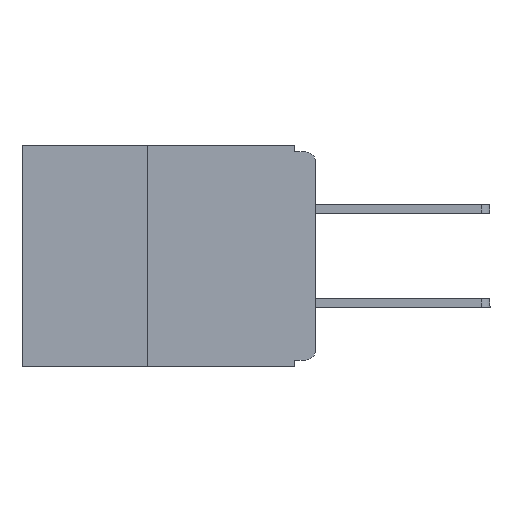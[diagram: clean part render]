
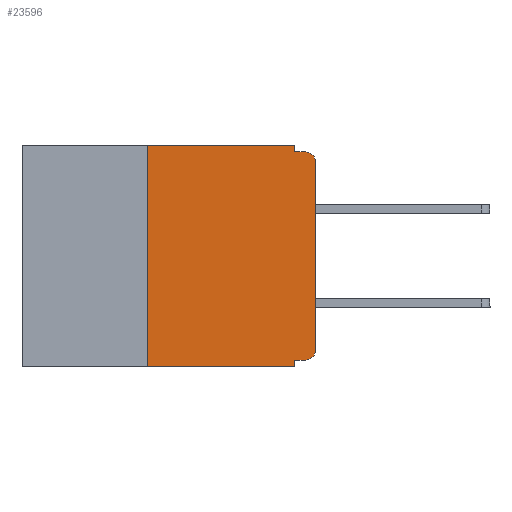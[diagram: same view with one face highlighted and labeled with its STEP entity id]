
A CAD part, left-side view. The second image highlights one B-rep face of the part: STEP entity #23596.
In plain terms, the highlighted planar face has unit normal (-1, 0, 0).
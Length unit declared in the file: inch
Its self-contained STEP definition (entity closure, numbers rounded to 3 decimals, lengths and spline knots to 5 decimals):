
#264 = EDGE_CURVE ( 'NONE', #24126, #7658, #23924, .T. ) ;
#312 = ORIENTED_EDGE ( 'NONE', *, *, #5832, .F. ) ;
#1313 = DIRECTION ( 'NONE',  ( 0., -1., 0. ) ) ;
#1519 = ORIENTED_EDGE ( 'NONE', *, *, #21155, .T. ) ;
#1641 = LINE ( 'NONE', #26766, #6741 ) ;
#2126 = EDGE_CURVE ( 'NONE', #22925, #6233, #27481, .T. ) ;
#2175 = ORIENTED_EDGE ( 'NONE', *, *, #25686, .F. ) ;
#2675 = CARTESIAN_POINT ( 'NONE',  ( 0., 0.015, -0.305 ) ) ;
#2694 = ORIENTED_EDGE ( 'NONE', *, *, #17311, .F. ) ;
#3103 = ORIENTED_EDGE ( 'NONE', *, *, #22706, .T. ) ;
#3152 = ORIENTED_EDGE ( 'NONE', *, *, #14555, .T. ) ;
#3421 = CARTESIAN_POINT ( 'NONE',  ( 0., 0., -0.305 ) ) ;
#3519 = CARTESIAN_POINT ( 'NONE',  ( 0., 0.031, -0.32 ) ) ;
#3711 = VERTEX_POINT ( 'NONE', #3519 ) ;
#4563 = DIRECTION ( 'NONE',  ( 0., 0., -1. ) ) ;
#4694 = CARTESIAN_POINT ( 'NONE',  ( 0., 0., -0.025 ) ) ;
#4832 = DIRECTION ( 'NONE',  ( 0., 0., -1. ) ) ;
#4986 = LINE ( 'NONE', #14463, #15992 ) ;
#5126 = ORIENTED_EDGE ( 'NONE', *, *, #20510, .F. ) ;
#5166 = VECTOR ( 'NONE', #14456, 39.37008 ) ;
#5707 = VECTOR ( 'NONE', #16219, 39.37008 ) ;
#5832 = EDGE_CURVE ( 'NONE', #23705, #10160, #15461, .T. ) ;
#6147 = CARTESIAN_POINT ( 'NONE',  ( 0., 0.25, -0.33 ) ) ;
#6233 = VERTEX_POINT ( 'NONE', #15600 ) ;
#6489 = VECTOR ( 'NONE', #25533, 39.37008 ) ;
#6550 = VERTEX_POINT ( 'NONE', #25217 ) ;
#6741 = VECTOR ( 'NONE', #18208, 39.37008 ) ;
#7175 = CARTESIAN_POINT ( 'NONE',  ( 0., 0.015, -0.025 ) ) ;
#7658 = VERTEX_POINT ( 'NONE', #4694 ) ;
#8170 = AXIS2_PLACEMENT_3D ( 'NONE', #2675, #17972, #4832 ) ;
#9197 = LINE ( 'NONE', #25203, #20206 ) ;
#9242 = CIRCLE ( 'NONE', #8170, 0.015 ) ;
#9347 = DIRECTION ( 'NONE',  ( 0., 0., -1. ) ) ;
#9460 = CARTESIAN_POINT ( 'NONE',  ( 0., 0.031, 0. ) ) ;
#9952 = CARTESIAN_POINT ( 'NONE',  ( 0., 0.031, 0. ) ) ;
#10160 = VERTEX_POINT ( 'NONE', #26424 ) ;
#10274 = VERTEX_POINT ( 'NONE', #9460 ) ;
#10350 = CARTESIAN_POINT ( 'NONE',  ( 0., 0.437, 0. ) ) ;
#10971 = LINE ( 'NONE', #9952, #5166 ) ;
#12144 = ORIENTED_EDGE ( 'NONE', *, *, #2126, .F. ) ;
#12612 = DIRECTION ( 'NONE',  ( 1., 0., 0. ) ) ;
#12910 = ORIENTED_EDGE ( 'NONE', *, *, #23468, .F. ) ;
#14456 = DIRECTION ( 'NONE',  ( 0., 0., -1. ) ) ;
#14463 = CARTESIAN_POINT ( 'NONE',  ( 0., 0.437, 0. ) ) ;
#14555 = EDGE_CURVE ( 'NONE', #6550, #24126, #9242, .T. ) ;
#14943 = VECTOR ( 'NONE', #4563, 39.37008 ) ;
#15448 = VERTEX_POINT ( 'NONE', #16599 ) ;
#15461 = LINE ( 'NONE', #24985, #26646 ) ;
#15600 = CARTESIAN_POINT ( 'NONE',  ( 0., 0.015, -0.01 ) ) ;
#15992 = VECTOR ( 'NONE', #1313, 39.37008 ) ;
#16219 = DIRECTION ( 'NONE',  ( 0., -1., 0. ) ) ;
#16599 = CARTESIAN_POINT ( 'NONE',  ( 0., 0.031, -0.33 ) ) ;
#16696 = CARTESIAN_POINT ( 'NONE',  ( 0., 0.031, -0.01 ) ) ;
#17311 = EDGE_CURVE ( 'NONE', #6550, #3711, #1641, .T. ) ;
#17972 = DIRECTION ( 'NONE',  ( -1., 0., 0. ) ) ;
#18208 = DIRECTION ( 'NONE',  ( 0., 1., 0. ) ) ;
#18287 = AXIS2_PLACEMENT_3D ( 'NONE', #10350, #12612, #27735 ) ;
#18366 = FACE_OUTER_BOUND ( 'NONE', #22217, .T. ) ;
#20206 = VECTOR ( 'NONE', #20957, 39.37008 ) ;
#20510 = EDGE_CURVE ( 'NONE', #10274, #22925, #10971, .T. ) ;
#20709 = LINE ( 'NONE', #26261, #14943 ) ;
#20957 = DIRECTION ( 'NONE',  ( 0., -1., 0. ) ) ;
#21155 = EDGE_CURVE ( 'NONE', #23705, #15448, #9197, .T. ) ;
#22217 = EDGE_LOOP ( 'NONE', ( #23411, #3103, #12144, #5126, #12910, #312, #1519, #2175, #2694, #3152 ) ) ;
#22454 = DIRECTION ( 'NONE',  ( -1., 0., 0. ) ) ;
#22706 = EDGE_CURVE ( 'NONE', #7658, #6233, #23463, .T. ) ;
#22925 = VERTEX_POINT ( 'NONE', #16696 ) ;
#23411 = ORIENTED_EDGE ( 'NONE', *, *, #264, .T. ) ;
#23446 = PLANE ( 'NONE',  #18287 ) ;
#23463 = CIRCLE ( 'NONE', #24775, 0.015 ) ;
#23468 = EDGE_CURVE ( 'NONE', #10160, #10274, #4986, .T. ) ;
#23596 = ADVANCED_FACE ( 'NONE', ( #18366 ), #23446, .F. ) ;
#23705 = VERTEX_POINT ( 'NONE', #6147 ) ;
#23924 = LINE ( 'NONE', #25525, #6489 ) ;
#24126 = VERTEX_POINT ( 'NONE', #3421 ) ;
#24775 = AXIS2_PLACEMENT_3D ( 'NONE', #7175, #22454, #9347 ) ;
#24985 = CARTESIAN_POINT ( 'NONE',  ( 0., 0.25, -0.33 ) ) ;
#25203 = CARTESIAN_POINT ( 'NONE',  ( 0., 0.437, -0.33 ) ) ;
#25217 = CARTESIAN_POINT ( 'NONE',  ( 0., 0.015, -0.32 ) ) ;
#25234 = CARTESIAN_POINT ( 'NONE',  ( 0., 0., -0.01 ) ) ;
#25525 = CARTESIAN_POINT ( 'NONE',  ( 0., 0., 0. ) ) ;
#25533 = DIRECTION ( 'NONE',  ( 0., 0., 1. ) ) ;
#25686 = EDGE_CURVE ( 'NONE', #3711, #15448, #20709, .T. ) ;
#26261 = CARTESIAN_POINT ( 'NONE',  ( 0., 0.031, -0.33 ) ) ;
#26424 = CARTESIAN_POINT ( 'NONE',  ( 0., 0.25, 0. ) ) ;
#26646 = VECTOR ( 'NONE', #27114, 39.37008 ) ;
#26766 = CARTESIAN_POINT ( 'NONE',  ( 0., 0., -0.32 ) ) ;
#27114 = DIRECTION ( 'NONE',  ( 0., 0., 1. ) ) ;
#27481 = LINE ( 'NONE', #25234, #5707 ) ;
#27735 = DIRECTION ( 'NONE',  ( 0., 0., -1. ) ) ;
